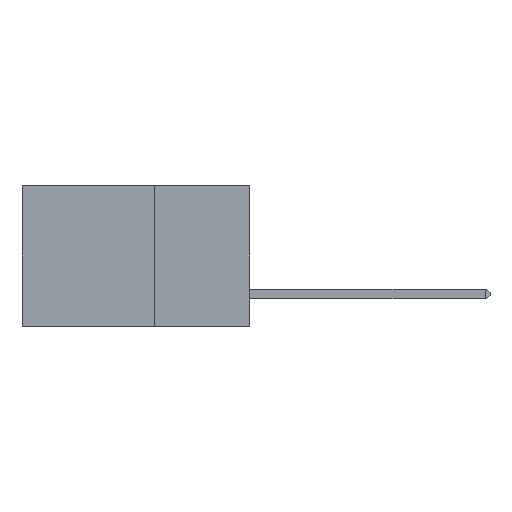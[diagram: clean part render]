
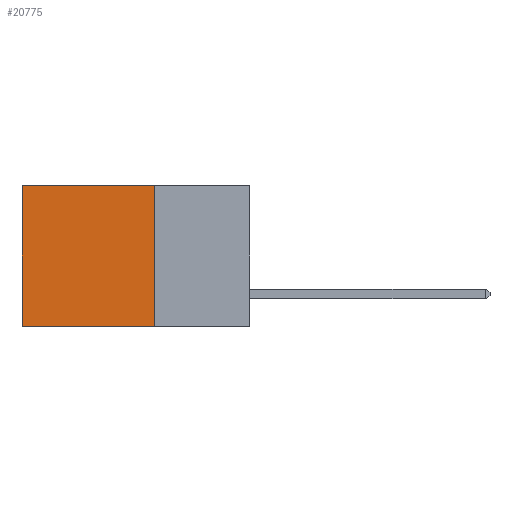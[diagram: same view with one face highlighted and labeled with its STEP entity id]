
A CAD part, left-side view. The second image highlights one B-rep face of the part: STEP entity #20775.
In plain terms, the highlighted planar face has unit normal (-1, 0, 0).
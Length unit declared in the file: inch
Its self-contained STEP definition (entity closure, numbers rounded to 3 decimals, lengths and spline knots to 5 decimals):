
#70 = CARTESIAN_POINT ( 'NONE',  ( 0.2875, 0.6, 0. ) ) ;
#510 = FACE_OUTER_BOUND ( 'NONE', #20325, .T. ) ;
#2052 = DIRECTION ( 'NONE',  ( 0., 1., 0. ) ) ;
#2054 = VECTOR ( 'NONE', #2052, 39.37008 ) ;
#3334 = PLANE ( 'NONE',  #28071 ) ;
#4924 = CARTESIAN_POINT ( 'NONE',  ( 0.2875, 0.25, -0.37 ) ) ;
#4994 = EDGE_CURVE ( 'NONE', #33003, #10213, #26558, .T. ) ;
#5955 = VECTOR ( 'NONE', #14720, 39.37008 ) ;
#8577 = DIRECTION ( 'NONE',  ( 1., 0., 0. ) ) ;
#8938 = VECTOR ( 'NONE', #31070, 39.37008 ) ;
#9606 = VERTEX_POINT ( 'NONE', #28128 ) ;
#10213 = VERTEX_POINT ( 'NONE', #4924 ) ;
#10595 = ORIENTED_EDGE ( 'NONE', *, *, #4994, .F. ) ;
#12103 = CARTESIAN_POINT ( 'NONE',  ( 0.2875, 0.25, 0. ) ) ;
#12448 = CARTESIAN_POINT ( 'NONE',  ( 0.2875, 0.25, -0.37 ) ) ;
#12881 = VECTOR ( 'NONE', #32892, 39.37008 ) ;
#12912 = CARTESIAN_POINT ( 'NONE',  ( 0.2875, 0.6, 0. ) ) ;
#14720 = DIRECTION ( 'NONE',  ( 0., 0., -1. ) ) ;
#15016 = CARTESIAN_POINT ( 'NONE',  ( 0.2875, 0.25, 0. ) ) ;
#15256 = ORIENTED_EDGE ( 'NONE', *, *, #25304, .T. ) ;
#16199 = EDGE_CURVE ( 'NONE', #10213, #9606, #23527, .T. ) ;
#17462 = EDGE_CURVE ( 'NONE', #29226, #9606, #30233, .T. ) ;
#20325 = EDGE_LOOP ( 'NONE', ( #21882, #23536, #10595, #15256 ) ) ;
#20775 = ADVANCED_FACE ( 'NONE', ( #510 ), #3334, .F. ) ;
#21882 = ORIENTED_EDGE ( 'NONE', *, *, #17462, .T. ) ;
#23527 = LINE ( 'NONE', #12448, #2054 ) ;
#23536 = ORIENTED_EDGE ( 'NONE', *, *, #16199, .F. ) ;
#24030 = CARTESIAN_POINT ( 'NONE',  ( 0.2875, 0.25, 0. ) ) ;
#25182 = CARTESIAN_POINT ( 'NONE',  ( 0.2875, 0.25, 0. ) ) ;
#25304 = EDGE_CURVE ( 'NONE', #33003, #29226, #32523, .T. ) ;
#26558 = LINE ( 'NONE', #12103, #5955 ) ;
#26605 = DIRECTION ( 'NONE',  ( 0., 0., -1. ) ) ;
#28071 = AXIS2_PLACEMENT_3D ( 'NONE', #24030, #8577, #26605 ) ;
#28128 = CARTESIAN_POINT ( 'NONE',  ( 0.2875, 0.6, -0.37 ) ) ;
#29226 = VERTEX_POINT ( 'NONE', #12912 ) ;
#30233 = LINE ( 'NONE', #70, #8938 ) ;
#31070 = DIRECTION ( 'NONE',  ( 0., 0., -1. ) ) ;
#32523 = LINE ( 'NONE', #15016, #12881 ) ;
#32892 = DIRECTION ( 'NONE',  ( 0., 1., 0. ) ) ;
#33003 = VERTEX_POINT ( 'NONE', #25182 ) ;
